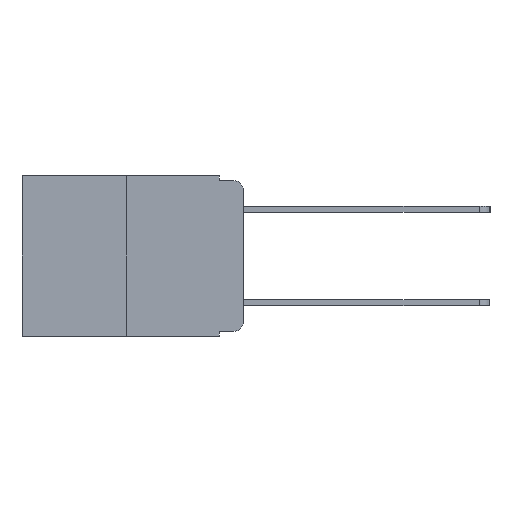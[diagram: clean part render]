
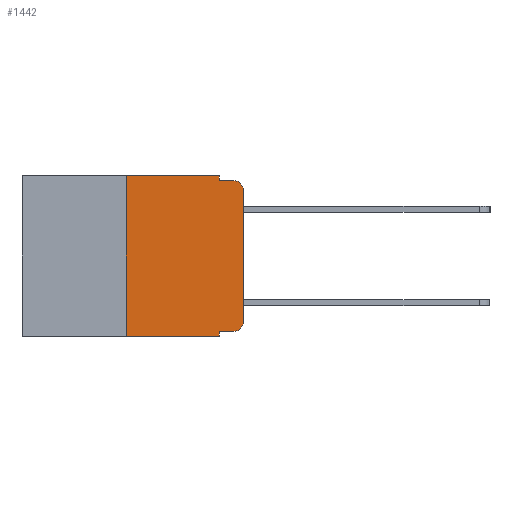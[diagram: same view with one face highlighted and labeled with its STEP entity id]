
A CAD part, left-side view. The second image highlights one B-rep face of the part: STEP entity #1442.
In plain terms, the highlighted planar face has unit normal (-1, 0, 0).
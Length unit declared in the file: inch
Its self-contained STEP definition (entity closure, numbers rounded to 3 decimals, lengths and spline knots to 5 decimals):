
#45 = DIRECTION ( 'NONE',  ( -1., 0., 0. ) ) ;
#991 = CARTESIAN_POINT ( 'NONE',  ( 0., 0.051, 0. ) ) ;
#1086 = VECTOR ( 'NONE', #15340, 39.37008 ) ;
#1222 = CIRCLE ( 'NONE', #5627, 0.02 ) ;
#1307 = DIRECTION ( 'NONE',  ( 0., 0., -1. ) ) ;
#1442 = ADVANCED_FACE ( 'NONE', ( #3645 ), #13962, .F. ) ;
#1835 = LINE ( 'NONE', #991, #5234 ) ;
#1891 = DIRECTION ( 'NONE',  ( 0., 0., 1. ) ) ;
#1959 = EDGE_CURVE ( 'NONE', #11879, #14771, #16270, .T. ) ;
#1975 = VERTEX_POINT ( 'NONE', #11938 ) ;
#2443 = VERTEX_POINT ( 'NONE', #15995 ) ;
#2947 = CARTESIAN_POINT ( 'NONE',  ( 0., 0.473, 0. ) ) ;
#2990 = EDGE_CURVE ( 'NONE', #6954, #11879, #8932, .T. ) ;
#3077 = CARTESIAN_POINT ( 'NONE',  ( 0., 0.02, -0.01 ) ) ;
#3325 = ORIENTED_EDGE ( 'NONE', *, *, #9221, .T. ) ;
#3398 = ORIENTED_EDGE ( 'NONE', *, *, #8387, .T. ) ;
#3645 = FACE_OUTER_BOUND ( 'NONE', #16561, .T. ) ;
#3653 = ORIENTED_EDGE ( 'NONE', *, *, #7526, .F. ) ;
#3670 = ORIENTED_EDGE ( 'NONE', *, *, #6665, .F. ) ;
#3717 = ORIENTED_EDGE ( 'NONE', *, *, #15071, .F. ) ;
#3734 = ORIENTED_EDGE ( 'NONE', *, *, #5797, .F. ) ;
#3818 = ORIENTED_EDGE ( 'NONE', *, *, #5143, .T. ) ;
#3852 = ORIENTED_EDGE ( 'NONE', *, *, #4912, .F. ) ;
#4037 = ORIENTED_EDGE ( 'NONE', *, *, #2990, .T. ) ;
#4136 = VECTOR ( 'NONE', #16887, 39.37008 ) ;
#4213 = ORIENTED_EDGE ( 'NONE', *, *, #1959, .T. ) ;
#4775 = CARTESIAN_POINT ( 'NONE',  ( 0., 0.051, -0.01 ) ) ;
#4912 = EDGE_CURVE ( 'NONE', #6954, #11463, #1835, .T. ) ;
#5143 = EDGE_CURVE ( 'NONE', #5735, #11463, #11005, .T. ) ;
#5234 = VECTOR ( 'NONE', #11027, 39.37008 ) ;
#5552 = VECTOR ( 'NONE', #1891, 39.37008 ) ;
#5627 = AXIS2_PLACEMENT_3D ( 'NONE', #6083, #14765, #7383 ) ;
#5735 = VERTEX_POINT ( 'NONE', #16985 ) ;
#5797 = EDGE_CURVE ( 'NONE', #5735, #2443, #13087, .T. ) ;
#6083 = CARTESIAN_POINT ( 'NONE',  ( 0., 0.02, -0.03 ) ) ;
#6172 = CARTESIAN_POINT ( 'NONE',  ( 0., 0., 0. ) ) ;
#6437 = LINE ( 'NONE', #2947, #13088 ) ;
#6665 = EDGE_CURVE ( 'NONE', #1975, #15435, #16886, .T. ) ;
#6954 = VERTEX_POINT ( 'NONE', #7631 ) ;
#7065 = DIRECTION ( 'NONE',  ( 0., 0., -1. ) ) ;
#7205 = LINE ( 'NONE', #4775, #10163 ) ;
#7383 = DIRECTION ( 'NONE',  ( 0., 0., -1. ) ) ;
#7526 = EDGE_CURVE ( 'NONE', #15435, #9717, #7205, .T. ) ;
#7631 = CARTESIAN_POINT ( 'NONE',  ( 0., 0.051, -0.333 ) ) ;
#8387 = EDGE_CURVE ( 'NONE', #9036, #9717, #1222, .T. ) ;
#8420 = CARTESIAN_POINT ( 'NONE',  ( 0., 0., -0.03 ) ) ;
#8932 = LINE ( 'NONE', #11986, #11861 ) ;
#9036 = VERTEX_POINT ( 'NONE', #8420 ) ;
#9083 = AXIS2_PLACEMENT_3D ( 'NONE', #15554, #15661, #7065 ) ;
#9221 = EDGE_CURVE ( 'NONE', #14771, #9036, #15467, .T. ) ;
#9717 = VERTEX_POINT ( 'NONE', #3077 ) ;
#10163 = VECTOR ( 'NONE', #12379, 39.37008 ) ;
#11005 = LINE ( 'NONE', #15360, #1086 ) ;
#11027 = DIRECTION ( 'NONE',  ( 0., 0., -1. ) ) ;
#11463 = VERTEX_POINT ( 'NONE', #16524 ) ;
#11539 = CARTESIAN_POINT ( 'NONE',  ( 0., 0., -0.313 ) ) ;
#11861 = VECTOR ( 'NONE', #11931, 39.37008 ) ;
#11879 = VERTEX_POINT ( 'NONE', #12524 ) ;
#11931 = DIRECTION ( 'NONE',  ( 0., -1., 0. ) ) ;
#11938 = CARTESIAN_POINT ( 'NONE',  ( 0., 0.051, 0. ) ) ;
#11986 = CARTESIAN_POINT ( 'NONE',  ( 0., 0.051, -0.333 ) ) ;
#12071 = DIRECTION ( 'NONE',  ( 0., -1., 0. ) ) ;
#12379 = DIRECTION ( 'NONE',  ( 0., -1., 0. ) ) ;
#12399 = CARTESIAN_POINT ( 'NONE',  ( 0., 0.051, 0. ) ) ;
#12469 = DIRECTION ( 'NONE',  ( 0., 0., -1. ) ) ;
#12524 = CARTESIAN_POINT ( 'NONE',  ( 0., 0.02, -0.333 ) ) ;
#12535 = CARTESIAN_POINT ( 'NONE',  ( 0., 0.051, -0.01 ) ) ;
#13087 = LINE ( 'NONE', #16290, #4136 ) ;
#13088 = VECTOR ( 'NONE', #12071, 39.37008 ) ;
#13634 = VECTOR ( 'NONE', #12469, 39.37008 ) ;
#13962 = PLANE ( 'NONE',  #9083 ) ;
#14765 = DIRECTION ( 'NONE',  ( -1., 0., 0. ) ) ;
#14771 = VERTEX_POINT ( 'NONE', #11539 ) ;
#14996 = CARTESIAN_POINT ( 'NONE',  ( 0., 0.02, -0.313 ) ) ;
#15071 = EDGE_CURVE ( 'NONE', #2443, #1975, #6437, .T. ) ;
#15340 = DIRECTION ( 'NONE',  ( 0., -1., 0. ) ) ;
#15360 = CARTESIAN_POINT ( 'NONE',  ( 0., 0.473, -0.343 ) ) ;
#15435 = VERTEX_POINT ( 'NONE', #12535 ) ;
#15467 = LINE ( 'NONE', #6172, #5552 ) ;
#15554 = CARTESIAN_POINT ( 'NONE',  ( 0., 0.473, 0. ) ) ;
#15661 = DIRECTION ( 'NONE',  ( 1., 0., 0. ) ) ;
#15874 = AXIS2_PLACEMENT_3D ( 'NONE', #14996, #45, #1307 ) ;
#15995 = CARTESIAN_POINT ( 'NONE',  ( 0., 0.25, 0. ) ) ;
#16270 = CIRCLE ( 'NONE', #15874, 0.02 ) ;
#16290 = CARTESIAN_POINT ( 'NONE',  ( 0., 0.25, 0. ) ) ;
#16524 = CARTESIAN_POINT ( 'NONE',  ( 0., 0.051, -0.343 ) ) ;
#16561 = EDGE_LOOP ( 'NONE', ( #3325, #3398, #3653, #3670, #3717, #3734, #3818, #3852, #4037, #4213 ) ) ;
#16886 = LINE ( 'NONE', #12399, #13634 ) ;
#16887 = DIRECTION ( 'NONE',  ( 0., 0., 1. ) ) ;
#16985 = CARTESIAN_POINT ( 'NONE',  ( 0., 0.25, -0.343 ) ) ;
